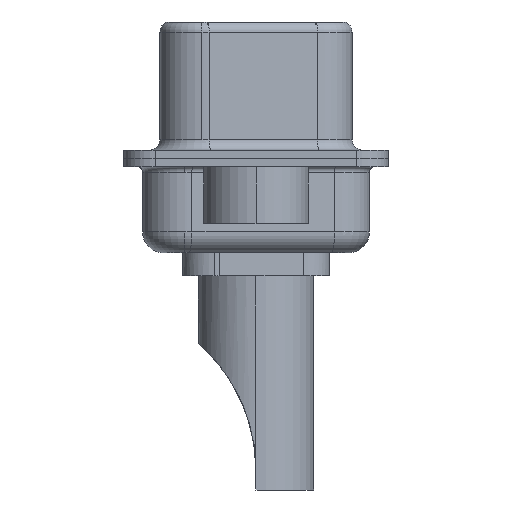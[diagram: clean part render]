
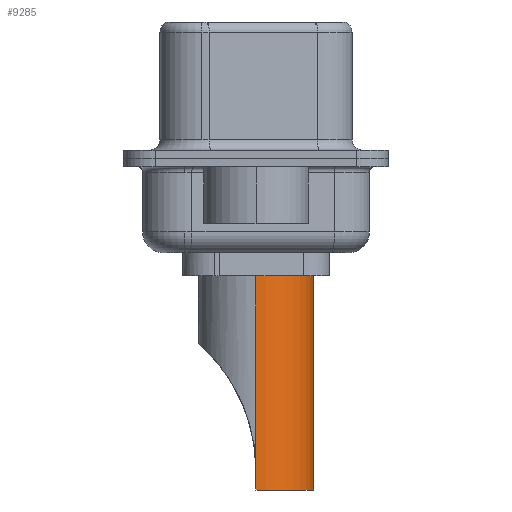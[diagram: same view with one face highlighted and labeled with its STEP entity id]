
A CAD part, left-side view. The second image highlights one B-rep face of the part: STEP entity #9285.
In plain terms, the highlighted cylindrical face has radius 2.75 mm (diameter 5.5 mm), a partial arc.
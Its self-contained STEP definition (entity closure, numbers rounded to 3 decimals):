
#243 = EDGE_CURVE ( 'NONE', #2188, #14221, #15688, .T. ) ;
#500 = CARTESIAN_POINT ( 'NONE',  ( -2.75, 0., 1.5 ) ) ;
#761 = DIRECTION ( 'NONE',  ( 0., 0., 1. ) ) ;
#1111 = LINE ( 'NONE', #13727, #14160 ) ;
#2188 = VERTEX_POINT ( 'NONE', #500 ) ;
#2215 = ORIENTED_EDGE ( 'NONE', *, *, #15461, .T. ) ;
#2364 = CARTESIAN_POINT ( 'NONE',  ( -2.75, 0., -8.7 ) ) ;
#2444 = DIRECTION ( 'NONE',  ( 1., 0., 0. ) ) ;
#2959 = DIRECTION ( 'NONE',  ( 1., 0., 0. ) ) ;
#3032 = AXIS2_PLACEMENT_3D ( 'NONE', #12759, #7653, #2959 ) ;
#3549 = DIRECTION ( 'NONE',  ( 0., 0., 1. ) ) ;
#5363 = ORIENTED_EDGE ( 'NONE', *, *, #20195, .F. ) ;
#5439 = DIRECTION ( 'NONE',  ( 0., 0., 1. ) ) ;
#6330 = AXIS2_PLACEMENT_3D ( 'NONE', #14370, #761, #2444 ) ;
#6595 = DIRECTION ( 'NONE',  ( 1., 0., 0. ) ) ;
#7063 = CARTESIAN_POINT ( 'NONE',  ( 2.75, 0., 4.234 ) ) ;
#7601 = VECTOR ( 'NONE', #12594, 1000. ) ;
#7653 = DIRECTION ( 'NONE',  ( 0., 0., 1. ) ) ;
#7722 = VERTEX_POINT ( 'NONE', #18640 ) ;
#9285 = ADVANCED_FACE ( 'NONE', ( #14674 ), #15454, .T. ) ;
#9338 = AXIS2_PLACEMENT_3D ( 'NONE', #16805, #3549, #6595 ) ;
#9736 = ORIENTED_EDGE ( 'NONE', *, *, #16874, .F. ) ;
#10151 = EDGE_CURVE ( 'NONE', #16847, #18330, #1111, .T. ) ;
#12111 = CARTESIAN_POINT ( 'NONE',  ( 2.75, 0., -8.7 ) ) ;
#12256 = CARTESIAN_POINT ( 'NONE',  ( 2.75, 0., -8.7 ) ) ;
#12409 = EDGE_LOOP ( 'NONE', ( #5363, #16795, #16625, #9736, #2215, #16835 ) ) ;
#12594 = DIRECTION ( 'NONE',  ( 0., 0., 1. ) ) ;
#12660 = CIRCLE ( 'NONE', #9338, 2.75 ) ;
#12759 = CARTESIAN_POINT ( 'NONE',  ( 0., 0., 4.234 ) ) ;
#12880 = LINE ( 'NONE', #7063, #13139 ) ;
#13139 = VECTOR ( 'NONE', #5439, 1000. ) ;
#13727 = CARTESIAN_POINT ( 'NONE',  ( -2.75, 0., -8.7 ) ) ;
#14160 = VECTOR ( 'NONE', #15519, 1000. ) ;
#14221 = VERTEX_POINT ( 'NONE', #16411 ) ;
#14292 = LINE ( 'NONE', #15840, #7601 ) ;
#14370 = CARTESIAN_POINT ( 'NONE',  ( 0., 0., 1.5 ) ) ;
#14378 = VERTEX_POINT ( 'NONE', #12111 ) ;
#14674 = FACE_OUTER_BOUND ( 'NONE', #12409, .T. ) ;
#15454 = CYLINDRICAL_SURFACE ( 'NONE', #3032, 2.75 ) ;
#15461 = EDGE_CURVE ( 'NONE', #7722, #14221, #12880, .T. ) ;
#15519 = DIRECTION ( 'NONE',  ( 0., 0., -1. ) ) ;
#15688 = CIRCLE ( 'NONE', #6330, 2.75 ) ;
#15840 = CARTESIAN_POINT ( 'NONE',  ( -2.75, 0., 4.234 ) ) ;
#16411 = CARTESIAN_POINT ( 'NONE',  ( 2.75, 0., 1.5 ) ) ;
#16548 = VECTOR ( 'NONE', #17380, 1000. ) ;
#16625 = ORIENTED_EDGE ( 'NONE', *, *, #21814, .T. ) ;
#16795 = ORIENTED_EDGE ( 'NONE', *, *, #10151, .T. ) ;
#16805 = CARTESIAN_POINT ( 'NONE',  ( 0., 0., -8.7 ) ) ;
#16835 = ORIENTED_EDGE ( 'NONE', *, *, #243, .F. ) ;
#16847 = VERTEX_POINT ( 'NONE', #20858 ) ;
#16874 = EDGE_CURVE ( 'NONE', #7722, #14378, #17341, .T. ) ;
#17341 = LINE ( 'NONE', #12256, #16548 ) ;
#17380 = DIRECTION ( 'NONE',  ( 0., 0., -1. ) ) ;
#18330 = VERTEX_POINT ( 'NONE', #2364 ) ;
#18640 = CARTESIAN_POINT ( 'NONE',  ( 2.75, 0., -7.764 ) ) ;
#20195 = EDGE_CURVE ( 'NONE', #16847, #2188, #14292, .T. ) ;
#20858 = CARTESIAN_POINT ( 'NONE',  ( -2.75, 0., -7.764 ) ) ;
#21814 = EDGE_CURVE ( 'NONE', #18330, #14378, #12660, .T. ) ;
